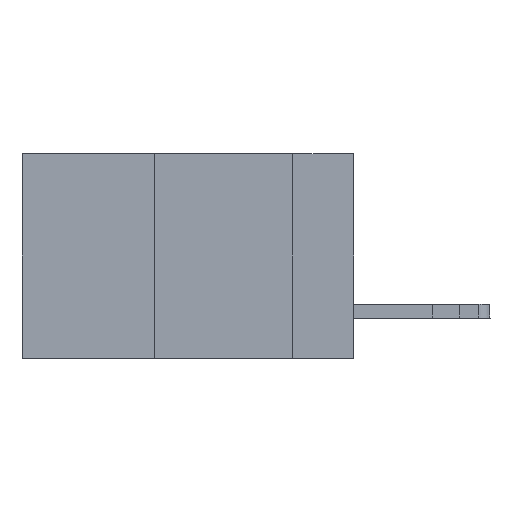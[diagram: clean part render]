
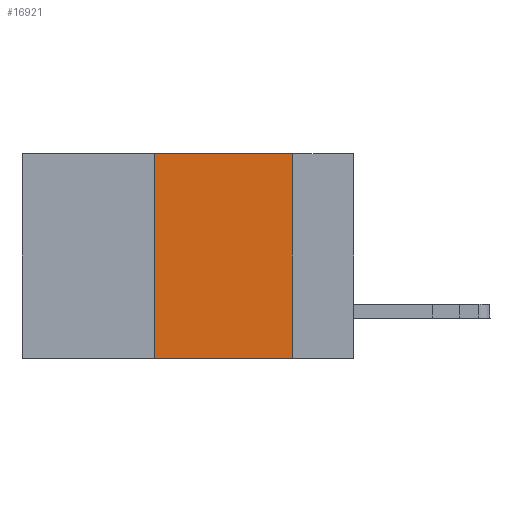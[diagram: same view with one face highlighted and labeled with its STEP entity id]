
A CAD part, left-side view. The second image highlights one B-rep face of the part: STEP entity #16921.
In plain terms, the highlighted planar face has unit normal (-1, 0, 0).
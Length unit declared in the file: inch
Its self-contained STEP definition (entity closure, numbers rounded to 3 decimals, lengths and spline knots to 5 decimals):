
#129 = ORIENTED_EDGE ( 'NONE', *, *, #25307, .T. ) ;
#365 = CARTESIAN_POINT ( 'NONE',  ( 0., 0.36, 0. ) ) ;
#2552 = CARTESIAN_POINT ( 'NONE',  ( 0., 0.11, 0. ) ) ;
#2924 = VERTEX_POINT ( 'NONE', #21626 ) ;
#3073 = ORIENTED_EDGE ( 'NONE', *, *, #17607, .F. ) ;
#4106 = VERTEX_POINT ( 'NONE', #14226 ) ;
#5226 = CARTESIAN_POINT ( 'NONE',  ( 0., 0.36, 0. ) ) ;
#5264 = CARTESIAN_POINT ( 'NONE',  ( 0., 0.6, 0. ) ) ;
#5320 = VERTEX_POINT ( 'NONE', #14667 ) ;
#5795 = EDGE_CURVE ( 'NONE', #21140, #2924, #22550, .T. ) ;
#7661 = DIRECTION ( 'NONE',  ( 0., -1., 0. ) ) ;
#9413 = DIRECTION ( 'NONE',  ( 0., 0., -1. ) ) ;
#10462 = AXIS2_PLACEMENT_3D ( 'NONE', #5264, #25972, #9413 ) ;
#10520 = LINE ( 'NONE', #26766, #26331 ) ;
#10952 = ORIENTED_EDGE ( 'NONE', *, *, #11562, .F. ) ;
#11253 = PLANE ( 'NONE',  #10462 ) ;
#11429 = LINE ( 'NONE', #2552, #21921 ) ;
#11562 = EDGE_CURVE ( 'NONE', #2924, #4106, #11429, .T. ) ;
#12142 = LINE ( 'NONE', #365, #15776 ) ;
#12386 = VECTOR ( 'NONE', #13990, 39.37008 ) ;
#13990 = DIRECTION ( 'NONE',  ( 0., -1., 0. ) ) ;
#14226 = CARTESIAN_POINT ( 'NONE',  ( 0., 0.11, -0.37 ) ) ;
#14667 = CARTESIAN_POINT ( 'NONE',  ( 0., 0.36, -0.37 ) ) ;
#14948 = DIRECTION ( 'NONE',  ( 0., 0., -1. ) ) ;
#15776 = VECTOR ( 'NONE', #26363, 39.37008 ) ;
#16374 = EDGE_LOOP ( 'NONE', ( #10952, #20663, #3073, #129 ) ) ;
#16921 = ADVANCED_FACE ( 'NONE', ( #23000 ), #11253, .F. ) ;
#17607 = EDGE_CURVE ( 'NONE', #5320, #21140, #12142, .T. ) ;
#20153 = CARTESIAN_POINT ( 'NONE',  ( 0., 0.6, 0. ) ) ;
#20663 = ORIENTED_EDGE ( 'NONE', *, *, #5795, .F. ) ;
#21140 = VERTEX_POINT ( 'NONE', #5226 ) ;
#21626 = CARTESIAN_POINT ( 'NONE',  ( 0., 0.11, 0. ) ) ;
#21921 = VECTOR ( 'NONE', #14948, 39.37008 ) ;
#22550 = LINE ( 'NONE', #20153, #12386 ) ;
#23000 = FACE_OUTER_BOUND ( 'NONE', #16374, .T. ) ;
#25307 = EDGE_CURVE ( 'NONE', #5320, #4106, #10520, .T. ) ;
#25972 = DIRECTION ( 'NONE',  ( 1., 0., 0. ) ) ;
#26331 = VECTOR ( 'NONE', #7661, 39.37008 ) ;
#26363 = DIRECTION ( 'NONE',  ( 0., 0., 1. ) ) ;
#26766 = CARTESIAN_POINT ( 'NONE',  ( 0., 0.6, -0.37 ) ) ;
